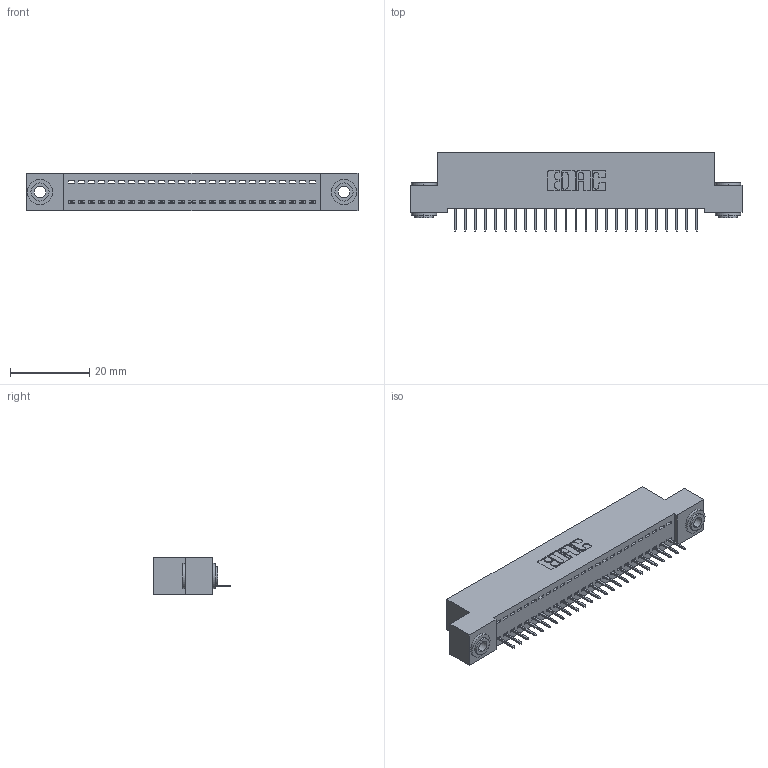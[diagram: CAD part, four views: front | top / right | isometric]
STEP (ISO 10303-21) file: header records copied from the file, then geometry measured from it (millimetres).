
FILE_DESCRIPTION (( 'STEP AP203' ), '1' );
FILE_NAME ('392-025-524-103.STEP', '2019-10-07T08:01:46', ( '' ), ( '' ), 'SwSTEP 2.0', 'SolidWorks 2016', '' );
FILE_SCHEMA (( 'CONFIG_CONTROL_DESIGN' ));
Length unit declared in the file: inch
Products named in the file (4): 342 Part_.156 TH; 345-292-001_345-293-124; 342-250-002_345-250-002-102; 392-025-524-103
Assembly tree (28 placements, depth 2):
  392-025-524-103
    342 Part_.156 TH
    345-292-001_345-293-124  x25
    342-250-002_345-250-002-102  x2
Bounding box: 83.82 x 19.69 x 9.4 mm (x, y, z)
Volume: 7210.8 mm3; surface area: 10190.7 mm2
Topology: 28 solids, 28 shells, 1698 faces, 4875 edges, 3146 vertices
Faces by surface type: plane 1276, cylinder 414, cone 8
Entity records: 18074 total; most frequent: CARTESIAN_POINT 3096, ORIENTED_EDGE 3050, DIRECTION 2681, EDGE_CURVE 1525, VECTOR 1377, LINE 1377, VERTEX_POINT 1010, AXIS2_PLACEMENT_3D 652
